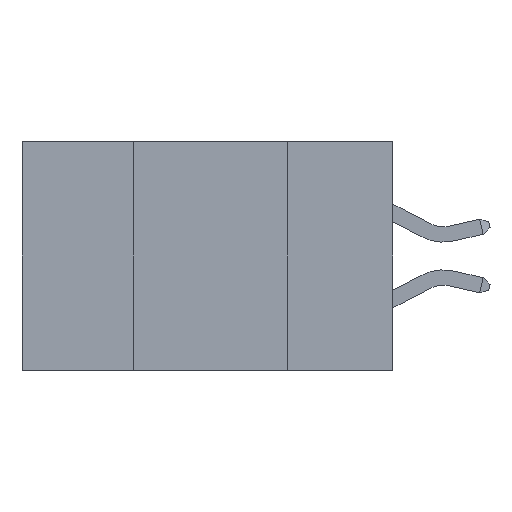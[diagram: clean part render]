
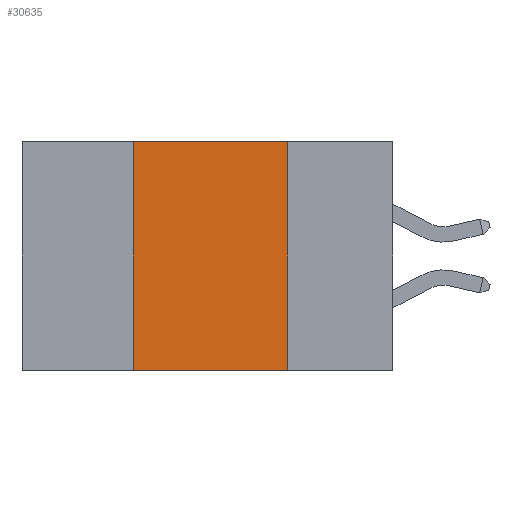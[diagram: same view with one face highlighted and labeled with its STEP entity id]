
A CAD part, left-side view. The second image highlights one B-rep face of the part: STEP entity #30635.
In plain terms, the highlighted planar face has unit normal (-1, 0, 0).
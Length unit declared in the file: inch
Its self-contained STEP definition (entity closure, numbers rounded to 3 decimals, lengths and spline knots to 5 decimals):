
#613 = VECTOR ( 'NONE', #25011, 39.37008 ) ;
#1204 = EDGE_CURVE ( 'NONE', #26210, #28261, #21507, .T. ) ;
#2699 = AXIS2_PLACEMENT_3D ( 'NONE', #22567, #12680, #29843 ) ;
#2773 = LINE ( 'NONE', #12157, #7857 ) ;
#3019 = EDGE_CURVE ( 'NONE', #28261, #7216, #3021, .T. ) ;
#3021 = LINE ( 'NONE', #26742, #15528 ) ;
#3102 = EDGE_CURVE ( 'NONE', #26210, #31187, #27051, .T. ) ;
#4599 = CARTESIAN_POINT ( 'NONE',  ( 0., 0.42, 0. ) ) ;
#5110 = CARTESIAN_POINT ( 'NONE',  ( 0., 0.17, -0.37 ) ) ;
#5130 = PLANE ( 'NONE',  #2699 ) ;
#7216 = VERTEX_POINT ( 'NONE', #30940 ) ;
#7857 = VECTOR ( 'NONE', #29346, 39.37008 ) ;
#7936 = EDGE_CURVE ( 'NONE', #7216, #31187, #2773, .T. ) ;
#12157 = CARTESIAN_POINT ( 'NONE',  ( 0., 0.17, 0. ) ) ;
#12680 = DIRECTION ( 'NONE',  ( 1., 0., 0. ) ) ;
#13079 = DIRECTION ( 'NONE',  ( 0., 0., 1. ) ) ;
#13801 = CARTESIAN_POINT ( 'NONE',  ( 0., 0.42, -0.37 ) ) ;
#14879 = VECTOR ( 'NONE', #13079, 39.37008 ) ;
#14974 = CARTESIAN_POINT ( 'NONE',  ( 0., 0.42, 0. ) ) ;
#15528 = VECTOR ( 'NONE', #28229, 39.37008 ) ;
#18820 = EDGE_LOOP ( 'NONE', ( #29439, #30604, #30186, #29600 ) ) ;
#19006 = FACE_OUTER_BOUND ( 'NONE', #18820, .T. ) ;
#21507 = LINE ( 'NONE', #14974, #14879 ) ;
#22567 = CARTESIAN_POINT ( 'NONE',  ( 0., 0.6, 0. ) ) ;
#25011 = DIRECTION ( 'NONE',  ( 0., -1., 0. ) ) ;
#26210 = VERTEX_POINT ( 'NONE', #13801 ) ;
#26742 = CARTESIAN_POINT ( 'NONE',  ( 0., 0.6, 0. ) ) ;
#27051 = LINE ( 'NONE', #27981, #613 ) ;
#27981 = CARTESIAN_POINT ( 'NONE',  ( 0., 0.6, -0.37 ) ) ;
#28229 = DIRECTION ( 'NONE',  ( 0., -1., 0. ) ) ;
#28261 = VERTEX_POINT ( 'NONE', #4599 ) ;
#29346 = DIRECTION ( 'NONE',  ( 0., 0., -1. ) ) ;
#29439 = ORIENTED_EDGE ( 'NONE', *, *, #7936, .F. ) ;
#29600 = ORIENTED_EDGE ( 'NONE', *, *, #3102, .T. ) ;
#29843 = DIRECTION ( 'NONE',  ( 0., 0., -1. ) ) ;
#30186 = ORIENTED_EDGE ( 'NONE', *, *, #1204, .F. ) ;
#30604 = ORIENTED_EDGE ( 'NONE', *, *, #3019, .F. ) ;
#30635 = ADVANCED_FACE ( 'NONE', ( #19006 ), #5130, .F. ) ;
#30940 = CARTESIAN_POINT ( 'NONE',  ( 0., 0.17, 0. ) ) ;
#31187 = VERTEX_POINT ( 'NONE', #5110 ) ;
